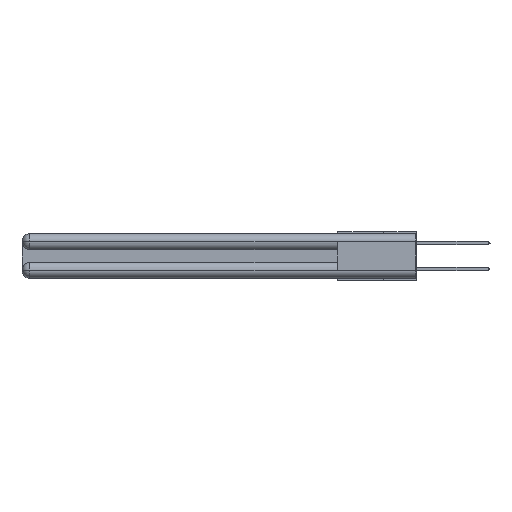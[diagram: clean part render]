
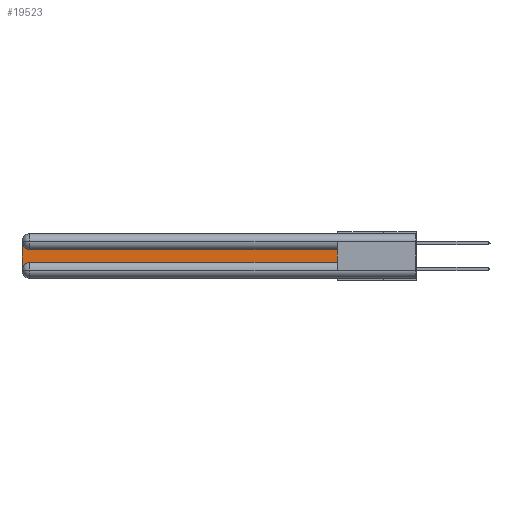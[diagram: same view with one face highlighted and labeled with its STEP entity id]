
A CAD part, left-side view. The second image highlights one B-rep face of the part: STEP entity #19523.
In plain terms, the highlighted planar face has unit normal (-1, 0, 0).
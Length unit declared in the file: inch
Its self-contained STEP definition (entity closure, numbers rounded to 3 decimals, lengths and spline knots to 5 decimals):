
#2019 = ORIENTED_EDGE ( 'NONE', *, *, #12894, .T. ) ;
#2103 = PLANE ( 'NONE',  #3230 ) ;
#2584 = CIRCLE ( 'NONE', #11004, 0.06 ) ;
#3201 = ORIENTED_EDGE ( 'NONE', *, *, #4409, .T. ) ;
#3230 = AXIS2_PLACEMENT_3D ( 'NONE', #26623, #15782, #21026 ) ;
#4082 = LINE ( 'NONE', #35340, #6685 ) ;
#4122 = ORIENTED_EDGE ( 'NONE', *, *, #33325, .T. ) ;
#4409 = EDGE_CURVE ( 'NONE', #29347, #13221, #11774, .T. ) ;
#4764 = VERTEX_POINT ( 'NONE', #24821 ) ;
#5194 = DIRECTION ( 'NONE',  ( 0., 1., 0. ) ) ;
#6685 = VECTOR ( 'NONE', #5194, 39.37008 ) ;
#7221 = VECTOR ( 'NONE', #17294, 39.37008 ) ;
#8985 = CARTESIAN_POINT ( 'NONE',  ( 0.075, 0.6, -0.2175 ) ) ;
#9146 = ORIENTED_EDGE ( 'NONE', *, *, #16504, .T. ) ;
#11004 = AXIS2_PLACEMENT_3D ( 'NONE', #17616, #20417, #18084 ) ;
#11774 = CIRCLE ( 'NONE', #33339, 0.06 ) ;
#12180 = CARTESIAN_POINT ( 'NONE',  ( 0.075, 3., -0.2175 ) ) ;
#12438 = CARTESIAN_POINT ( 'NONE',  ( 0.075, 0.6, -0.1225 ) ) ;
#12474 = LINE ( 'NONE', #12180, #7221 ) ;
#12894 = EDGE_CURVE ( 'NONE', #4764, #21282, #2584, .T. ) ;
#12965 = CARTESIAN_POINT ( 'NONE',  ( 0.075, 0.6, -0.2175 ) ) ;
#13221 = VERTEX_POINT ( 'NONE', #28140 ) ;
#13733 = EDGE_LOOP ( 'NONE', ( #32325, #2019, #4122, #3201, #27784, #9146 ) ) ;
#15782 = DIRECTION ( 'NONE',  ( 1., 0., 0. ) ) ;
#16504 = EDGE_CURVE ( 'NONE', #16912, #22219, #35439, .T. ) ;
#16912 = VERTEX_POINT ( 'NONE', #8985 ) ;
#17294 = DIRECTION ( 'NONE',  ( 0., 0., -1. ) ) ;
#17616 = CARTESIAN_POINT ( 'NONE',  ( 0.075, 2.94, -0.0625 ) ) ;
#18084 = DIRECTION ( 'NONE',  ( 0., 0., -1. ) ) ;
#18823 = EDGE_CURVE ( 'NONE', #13221, #16912, #19302, .T. ) ;
#18880 = EDGE_CURVE ( 'NONE', #22219, #4764, #4082, .T. ) ;
#19302 = LINE ( 'NONE', #12965, #24062 ) ;
#19523 = ADVANCED_FACE ( 'NONE', ( #26624 ), #2103, .F. ) ;
#19589 = CARTESIAN_POINT ( 'NONE',  ( 0.075, 3., -0.2775 ) ) ;
#20417 = DIRECTION ( 'NONE',  ( 1., 0., 0. ) ) ;
#21026 = DIRECTION ( 'NONE',  ( 0., 0., -1. ) ) ;
#21282 = VERTEX_POINT ( 'NONE', #34101 ) ;
#21580 = CARTESIAN_POINT ( 'NONE',  ( 0.075, 2.94, -0.2775 ) ) ;
#22219 = VERTEX_POINT ( 'NONE', #12438 ) ;
#22562 = DIRECTION ( 'NONE',  ( 0., 0., 1. ) ) ;
#22879 = VECTOR ( 'NONE', #22562, 39.37008 ) ;
#23980 = DIRECTION ( 'NONE',  ( 0., -1., 0. ) ) ;
#24062 = VECTOR ( 'NONE', #23980, 39.37008 ) ;
#24821 = CARTESIAN_POINT ( 'NONE',  ( 0.075, 2.94, -0.1225 ) ) ;
#26623 = CARTESIAN_POINT ( 'NONE',  ( 0.075, 3., -0.1225 ) ) ;
#26624 = FACE_OUTER_BOUND ( 'NONE', #13733, .T. ) ;
#27409 = DIRECTION ( 'NONE',  ( 1., 0., 0. ) ) ;
#27784 = ORIENTED_EDGE ( 'NONE', *, *, #18823, .T. ) ;
#28140 = CARTESIAN_POINT ( 'NONE',  ( 0.075, 2.94, -0.2175 ) ) ;
#29347 = VERTEX_POINT ( 'NONE', #19589 ) ;
#29674 = DIRECTION ( 'NONE',  ( 0., 0., -1. ) ) ;
#30173 = CARTESIAN_POINT ( 'NONE',  ( 0.075, 0.6, -0.2175 ) ) ;
#32325 = ORIENTED_EDGE ( 'NONE', *, *, #18880, .T. ) ;
#33325 = EDGE_CURVE ( 'NONE', #21282, #29347, #12474, .T. ) ;
#33339 = AXIS2_PLACEMENT_3D ( 'NONE', #21580, #27409, #29674 ) ;
#34101 = CARTESIAN_POINT ( 'NONE',  ( 0.075, 3., -0.0625 ) ) ;
#35340 = CARTESIAN_POINT ( 'NONE',  ( 0.075, 0.6, -0.1225 ) ) ;
#35439 = LINE ( 'NONE', #30173, #22879 ) ;
